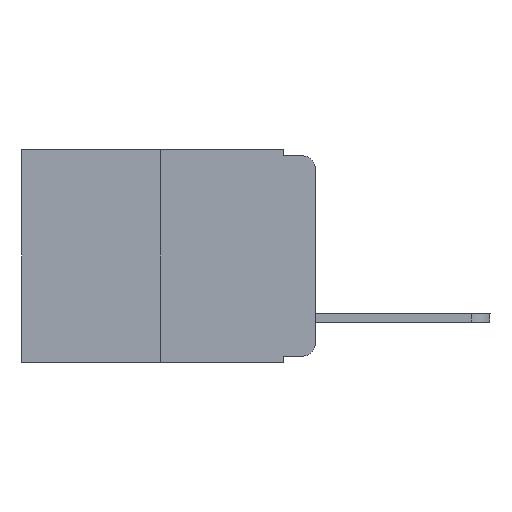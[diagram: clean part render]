
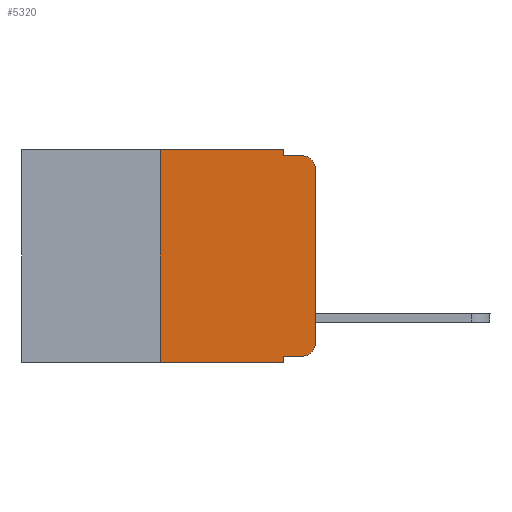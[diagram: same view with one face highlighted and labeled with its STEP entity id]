
A CAD part, left-side view. The second image highlights one B-rep face of the part: STEP entity #5320.
In plain terms, the highlighted planar face has unit normal (-1, 0, 0).
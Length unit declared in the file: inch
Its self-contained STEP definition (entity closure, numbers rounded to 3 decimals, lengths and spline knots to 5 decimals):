
#18 = CARTESIAN_POINT ( 'NONE',  ( 0., 0.02, -0.03 ) ) ;
#175 = CARTESIAN_POINT ( 'NONE',  ( 0., 0.02, -0.333 ) ) ;
#432 = EDGE_CURVE ( 'NONE', #3607, #1996, #613, .T. ) ;
#584 = FACE_OUTER_BOUND ( 'NONE', #7251, .T. ) ;
#599 = CARTESIAN_POINT ( 'NONE',  ( 0., 0., -0.313 ) ) ;
#613 = CIRCLE ( 'NONE', #6462, 0.02 ) ;
#712 = CARTESIAN_POINT ( 'NONE',  ( 0., 0.051, -0.333 ) ) ;
#715 = CARTESIAN_POINT ( 'NONE',  ( 0., 0.051, 0. ) ) ;
#827 = CARTESIAN_POINT ( 'NONE',  ( 0., 0.25, -0.343 ) ) ;
#1098 = VERTEX_POINT ( 'NONE', #827 ) ;
#1129 = ORIENTED_EDGE ( 'NONE', *, *, #7885, .T. ) ;
#1133 = CARTESIAN_POINT ( 'NONE',  ( 0., 0.051, 0. ) ) ;
#1265 = DIRECTION ( 'NONE',  ( 0., 0., -1. ) ) ;
#1441 = DIRECTION ( 'NONE',  ( 0., 0., -1. ) ) ;
#1447 = ORIENTED_EDGE ( 'NONE', *, *, #5696, .F. ) ;
#1475 = CARTESIAN_POINT ( 'NONE',  ( 0., 0.02, -0.01 ) ) ;
#1521 = DIRECTION ( 'NONE',  ( 0., 0., -1. ) ) ;
#1623 = EDGE_CURVE ( 'NONE', #1098, #9450, #3598, .T. ) ;
#1671 = CARTESIAN_POINT ( 'NONE',  ( 0., 0.051, -0.343 ) ) ;
#1832 = VECTOR ( 'NONE', #5103, 39.37008 ) ;
#1988 = DIRECTION ( 'NONE',  ( 1., 0., 0. ) ) ;
#1996 = VERTEX_POINT ( 'NONE', #1475 ) ;
#2378 = VERTEX_POINT ( 'NONE', #1133 ) ;
#2604 = EDGE_CURVE ( 'NONE', #9450, #2378, #6882, .T. ) ;
#2632 = EDGE_CURVE ( 'NONE', #4964, #3607, #4448, .T. ) ;
#2742 = LINE ( 'NONE', #5731, #1832 ) ;
#2755 = CARTESIAN_POINT ( 'NONE',  ( 0., 0.473, 0. ) ) ;
#2781 = CARTESIAN_POINT ( 'NONE',  ( 0., 0.25, 0. ) ) ;
#2849 = EDGE_CURVE ( 'NONE', #4745, #4964, #3162, .T. ) ;
#2877 = ORIENTED_EDGE ( 'NONE', *, *, #1623, .F. ) ;
#2890 = LINE ( 'NONE', #6594, #8419 ) ;
#2933 = EDGE_CURVE ( 'NONE', #2378, #8926, #2890, .T. ) ;
#2967 = DIRECTION ( 'NONE',  ( -1., 0., 0. ) ) ;
#3156 = CARTESIAN_POINT ( 'NONE',  ( 0., 0.473, -0.343 ) ) ;
#3160 = CARTESIAN_POINT ( 'NONE',  ( 0., 0.051, -0.01 ) ) ;
#3162 = CIRCLE ( 'NONE', #4395, 0.02 ) ;
#3243 = VECTOR ( 'NONE', #9448, 39.37008 ) ;
#3321 = VERTEX_POINT ( 'NONE', #712 ) ;
#3598 = LINE ( 'NONE', #8733, #8863 ) ;
#3607 = VERTEX_POINT ( 'NONE', #6367 ) ;
#3659 = ORIENTED_EDGE ( 'NONE', *, *, #9484, .F. ) ;
#4046 = CARTESIAN_POINT ( 'NONE',  ( 0., 0.473, 0. ) ) ;
#4395 = AXIS2_PLACEMENT_3D ( 'NONE', #6687, #7359, #1441 ) ;
#4448 = LINE ( 'NONE', #5945, #7813 ) ;
#4696 = VECTOR ( 'NONE', #5094, 39.37008 ) ;
#4745 = VERTEX_POINT ( 'NONE', #175 ) ;
#4830 = LINE ( 'NONE', #9401, #3243 ) ;
#4964 = VERTEX_POINT ( 'NONE', #599 ) ;
#5051 = ORIENTED_EDGE ( 'NONE', *, *, #2632, .T. ) ;
#5094 = DIRECTION ( 'NONE',  ( 0., 0., -1. ) ) ;
#5103 = DIRECTION ( 'NONE',  ( 0., -1., 0. ) ) ;
#5320 = ADVANCED_FACE ( 'NONE', ( #584 ), #5741, .F. ) ;
#5503 = DIRECTION ( 'NONE',  ( 0., -1., 0. ) ) ;
#5669 = ORIENTED_EDGE ( 'NONE', *, *, #432, .T. ) ;
#5696 = EDGE_CURVE ( 'NONE', #8926, #1996, #2742, .T. ) ;
#5731 = CARTESIAN_POINT ( 'NONE',  ( 0., 0.051, -0.01 ) ) ;
#5741 = PLANE ( 'NONE',  #8008 ) ;
#5945 = CARTESIAN_POINT ( 'NONE',  ( 0., 0., 0. ) ) ;
#6256 = DIRECTION ( 'NONE',  ( 0., -1., 0. ) ) ;
#6257 = ORIENTED_EDGE ( 'NONE', *, *, #2604, .F. ) ;
#6367 = CARTESIAN_POINT ( 'NONE',  ( 0., 0., -0.03 ) ) ;
#6462 = AXIS2_PLACEMENT_3D ( 'NONE', #18, #2967, #1521 ) ;
#6594 = CARTESIAN_POINT ( 'NONE',  ( 0., 0.051, 0. ) ) ;
#6687 = CARTESIAN_POINT ( 'NONE',  ( 0., 0.02, -0.313 ) ) ;
#6783 = VECTOR ( 'NONE', #5503, 39.37008 ) ;
#6841 = ORIENTED_EDGE ( 'NONE', *, *, #2849, .T. ) ;
#6882 = LINE ( 'NONE', #4046, #8141 ) ;
#7251 = EDGE_LOOP ( 'NONE', ( #5051, #5669, #1447, #8883, #6257, #2877, #1129, #3659, #8697, #6841 ) ) ;
#7359 = DIRECTION ( 'NONE',  ( -1., 0., 0. ) ) ;
#7434 = DIRECTION ( 'NONE',  ( 0., 0., 1. ) ) ;
#7676 = VERTEX_POINT ( 'NONE', #1671 ) ;
#7813 = VECTOR ( 'NONE', #7434, 39.37008 ) ;
#7885 = EDGE_CURVE ( 'NONE', #1098, #7676, #9214, .T. ) ;
#7996 = EDGE_CURVE ( 'NONE', #3321, #4745, #4830, .T. ) ;
#8008 = AXIS2_PLACEMENT_3D ( 'NONE', #2755, #1988, #1265 ) ;
#8141 = VECTOR ( 'NONE', #6256, 39.37008 ) ;
#8208 = LINE ( 'NONE', #715, #4696 ) ;
#8419 = VECTOR ( 'NONE', #8833, 39.37008 ) ;
#8697 = ORIENTED_EDGE ( 'NONE', *, *, #7996, .T. ) ;
#8733 = CARTESIAN_POINT ( 'NONE',  ( 0., 0.25, 0. ) ) ;
#8833 = DIRECTION ( 'NONE',  ( 0., 0., -1. ) ) ;
#8863 = VECTOR ( 'NONE', #9514, 39.37008 ) ;
#8883 = ORIENTED_EDGE ( 'NONE', *, *, #2933, .F. ) ;
#8926 = VERTEX_POINT ( 'NONE', #3160 ) ;
#9214 = LINE ( 'NONE', #3156, #6783 ) ;
#9401 = CARTESIAN_POINT ( 'NONE',  ( 0., 0.051, -0.333 ) ) ;
#9448 = DIRECTION ( 'NONE',  ( 0., -1., 0. ) ) ;
#9450 = VERTEX_POINT ( 'NONE', #2781 ) ;
#9484 = EDGE_CURVE ( 'NONE', #3321, #7676, #8208, .T. ) ;
#9514 = DIRECTION ( 'NONE',  ( 0., 0., 1. ) ) ;
